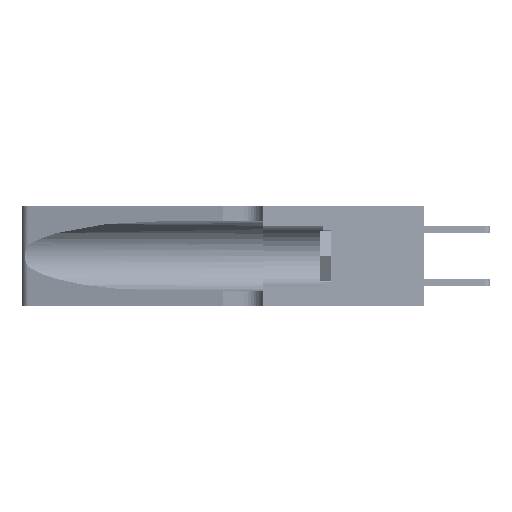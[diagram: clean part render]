
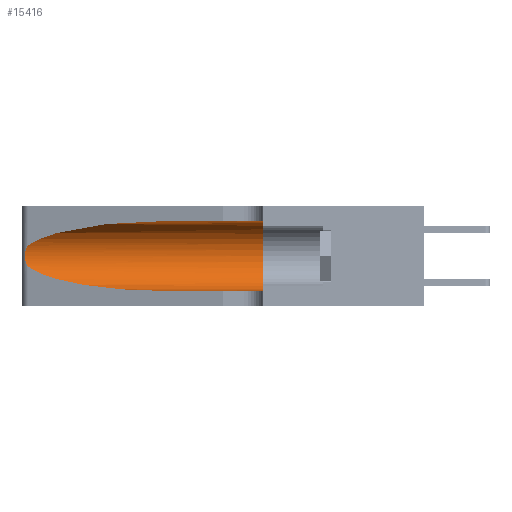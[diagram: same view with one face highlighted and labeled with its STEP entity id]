
A CAD part, left-side view. The second image highlights one B-rep face of the part: STEP entity #15416.
In plain terms, the highlighted cylindrical face has radius 3.308 mm (diameter 6.617 mm), a partial arc.
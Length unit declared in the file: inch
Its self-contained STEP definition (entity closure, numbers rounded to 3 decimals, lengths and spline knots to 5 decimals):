
#35 = CARTESIAN_POINT ( 'NONE',  ( 0.25856, 1.23593, 0.16098 ) ) ;
#537 = ORIENTED_EDGE ( 'NONE', *, *, #38185, .T. ) ;
#1724 = CARTESIAN_POINT ( 'NONE',  ( 0.25487, 1.22718, 0.14631 ) ) ;
#4579 = DIRECTION ( 'NONE',  ( 0., 1., 0. ) ) ;
#5739 = AXIS2_PLACEMENT_3D ( 'NONE', #36601, #17236, #48951 ) ;
#5752 = LINE ( 'NONE', #25447, #18096 ) ;
#6017 = VERTEX_POINT ( 'NONE', #16034 ) ;
#6989 = CARTESIAN_POINT ( 'NONE',  ( 0.1305, 0.35, 0.31525 ) ) ;
#7025 = AXIS2_PLACEMENT_3D ( 'NONE', #27922, #4579, #43696 ) ;
#7654 = CARTESIAN_POINT ( 'NONE',  ( 0.25639, 1.23184, 0.21858 ) ) ;
#7982 = CARTESIAN_POINT ( 'NONE',  ( 0.26075, 1.23896, 0.19203 ) ) ;
#8994 = CARTESIAN_POINT ( 'NONE',  ( 0.1305, 0.72297, 0.05475 ) ) ;
#9487 = ORIENTED_EDGE ( 'NONE', *, *, #45115, .T. ) ;
#9679 = CARTESIAN_POINT ( 'NONE',  ( 0.2373, 1.15595, 0.08982 ) ) ;
#9746 = VERTEX_POINT ( 'NONE', #9936 ) ;
#9936 = CARTESIAN_POINT ( 'NONE',  ( 0.1305, 0.72297, 0.05475 ) ) ;
#10180 = CARTESIAN_POINT ( 'NONE',  ( 0.1305, 0.72297, 0.31525 ) ) ;
#13335 = DIRECTION ( 'NONE',  ( 0., -1., 0. ) ) ;
#13764 = EDGE_CURVE ( 'NONE', #35639, #6017, #35324, .T. ) ;
#13913 = DIRECTION ( 'NONE',  ( 0., -1., 0. ) ) ;
#14247 = VERTEX_POINT ( 'NONE', #26683 ) ;
#14704 = CARTESIAN_POINT ( 'NONE',  ( 0.25487, 1.22718, 0.14631 ) ) ;
#15416 = ADVANCED_FACE ( 'NONE', ( #20642 ), #16950, .F. ) ;
#15805 = CARTESIAN_POINT ( 'NONE',  ( 0.1305, 0.72297, 0.31525 ) ) ;
#16034 = CARTESIAN_POINT ( 'NONE',  ( 0.1305, 0.35, 0.05475 ) ) ;
#16099 = CARTESIAN_POINT ( 'NONE',  ( 0.26018, 1.23835, 0.19895 ) ) ;
#16950 = CYLINDRICAL_SURFACE ( 'NONE', #5739, 0.13025 ) ;
#17236 = DIRECTION ( 'NONE',  ( 0., -1., 0. ) ) ;
#17940 = CARTESIAN_POINT ( 'NONE',  ( 0.2373, 1.15595, 0.28018 ) ) ;
#18096 = VECTOR ( 'NONE', #13335, 39.37008 ) ;
#19716 = CARTESIAN_POINT ( 'NONE',  ( 0.25639, 1.23186, 0.15144 ) ) ;
#20250 = ORIENTED_EDGE ( 'NONE', *, *, #41837, .F. ) ;
#20642 = FACE_OUTER_BOUND ( 'NONE', #29672, .T. ) ;
#22904 = ORIENTED_EDGE ( 'NONE', *, *, #41154, .T. ) ;
#23361 = CARTESIAN_POINT ( 'NONE',  ( 0.25555, 1.22993, 0.14849 ) ) ;
#23546 = CARTESIAN_POINT ( 'NONE',  ( 0.25487, 1.22718, 0.14631 ) ) ;
#23724 = CARTESIAN_POINT ( 'NONE',  ( 0.25854, 1.2359, 0.20912 ) ) ;
#24525 = EDGE_CURVE ( 'NONE', #9746, #6017, #5752, .T. ) ;
#25016 = CARTESIAN_POINT ( 'NONE',  ( 0.1305, 1.61858, 0.31525 ) ) ;
#25238 = VERTEX_POINT ( 'NONE', #15805 ) ;
#25447 = CARTESIAN_POINT ( 'NONE',  ( 0.1305, 1.61858, 0.05475 ) ) ;
#26683 = CARTESIAN_POINT ( 'NONE',  ( 0.25487, 1.22718, 0.22369 ) ) ;
#27347 = CARTESIAN_POINT ( 'NONE',  ( 0.25555, 1.22994, 0.2215 ) ) ;
#27514 = CARTESIAN_POINT ( 'NONE',  ( 0.25487, 1.22718, 0.22369 ) ) ;
#27922 = CARTESIAN_POINT ( 'NONE',  ( 0.1305, 0.35, 0.185 ) ) ;
#29672 = EDGE_LOOP ( 'NONE', ( #9487, #537, #22904, #37992, #33769, #20250 ) ) ;
#32674 = CARTESIAN_POINT ( 'NONE',  ( 0.18966, 0.96281, 0.05475 ) ) ;
#33769 = ORIENTED_EDGE ( 'NONE', *, *, #13764, .F. ) ;
#35300 = CARTESIAN_POINT ( 'NONE',  ( 0.26017, 1.23833, 0.17102 ) ) ;
#35324 = CIRCLE ( 'NONE', #7025, 0.13025 ) ;
#35639 = VERTEX_POINT ( 'NONE', #6989 ) ;
#36456 = LINE ( 'NONE', #25016, #42703 ) ;
#36601 = CARTESIAN_POINT ( 'NONE',  ( 0.1305, 1.61858, 0.185 ) ) ;
#37657 = CARTESIAN_POINT ( 'NONE',  ( 0.25487, 1.22718, 0.22369 ) ) ;
#37838 = CARTESIAN_POINT ( 'NONE',  ( 0.18966, 0.96281, 0.31525 ) ) ;
#37992 = ORIENTED_EDGE ( 'NONE', *, *, #24525, .T. ) ;
#38185 = EDGE_CURVE ( 'NONE', #14247, #40660, #46905, .T. ) ;
#39116 = CARTESIAN_POINT ( 'NONE',  ( 0.25787, 1.23484, 0.2124 ) ) ;
#39813 = CARTESIAN_POINT ( 'NONE',  ( 0.25789, 1.23486, 0.15765 ) ) ;
#40660 = VERTEX_POINT ( 'NONE', #14704 ) ;
#41154 = EDGE_CURVE ( 'NONE', #40660, #9746, #41493, .T. ) ;
#41493 =( BOUNDED_CURVE ( )  B_SPLINE_CURVE ( 3, ( #1724, #9679, #32674, #8994 ),
 .UNSPECIFIED., .F., .F. ) 
 B_SPLINE_CURVE_WITH_KNOTS ( ( 4, 4 ),
 ( 3.44316, 4.71239 ),
 .UNSPECIFIED. ) 
 CURVE ( )  GEOMETRIC_REPRESENTATION_ITEM ( )  RATIONAL_B_SPLINE_CURVE ( ( 1., 0.87, 0.87, 1. ) ) 
 REPRESENTATION_ITEM ( '' )  );
#41837 = EDGE_CURVE ( 'NONE', #25238, #35639, #36456, .T. ) ;
#42703 = VECTOR ( 'NONE', #13913, 39.37008 ) ;
#43696 = DIRECTION ( 'NONE',  ( 0., 0., 1. ) ) ;
#45115 = EDGE_CURVE ( 'NONE', #25238, #14247, #45969, .T. ) ;
#45969 =( BOUNDED_CURVE ( )  B_SPLINE_CURVE ( 3, ( #10180, #37838, #17940, #37657 ),
 .UNSPECIFIED., .F., .F. ) 
 B_SPLINE_CURVE_WITH_KNOTS ( ( 4, 4 ),
 ( 1.5708, 2.84003 ),
 .UNSPECIFIED. ) 
 CURVE ( )  GEOMETRIC_REPRESENTATION_ITEM ( )  RATIONAL_B_SPLINE_CURVE ( ( 1., 0.87, 0.87, 1. ) ) 
 REPRESENTATION_ITEM ( '' )  );
#46905 = B_SPLINE_CURVE_WITH_KNOTS ( 'NONE', 3,
 ( #27514, #27347, #7654, #39116, #23724, #16099, #7982, #47125, #35300, #35, #39813, #19716, #23361, #23546 ),
 .UNSPECIFIED., .F., .F.,
 ( 4, 2, 2, 2, 2, 2, 4 ),
 ( 0., 0.00027, 0.00053, 0.00107, 0.0016, 0.00187, 0.00214 ),
 .UNSPECIFIED. ) ;
#47125 = CARTESIAN_POINT ( 'NONE',  ( 0.26075, 1.23896, 0.178 ) ) ;
#48951 = DIRECTION ( 'NONE',  ( 0., 0., -1. ) ) ;
